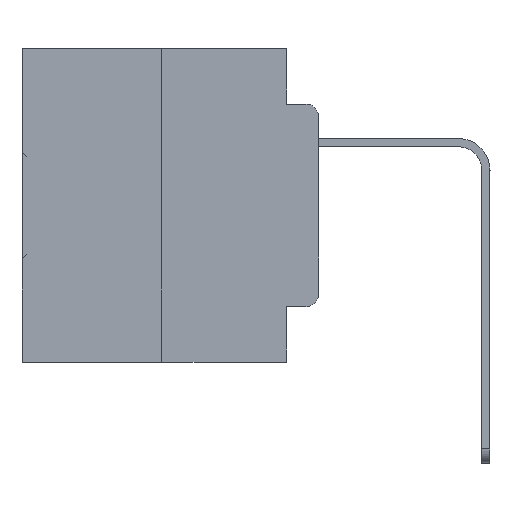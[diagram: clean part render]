
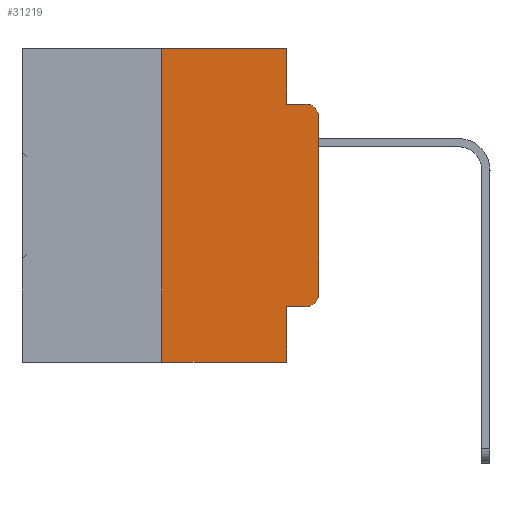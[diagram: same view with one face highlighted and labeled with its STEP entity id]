
A CAD part, left-side view. The second image highlights one B-rep face of the part: STEP entity #31219.
In plain terms, the highlighted planar face has unit normal (-1, 0, 0).
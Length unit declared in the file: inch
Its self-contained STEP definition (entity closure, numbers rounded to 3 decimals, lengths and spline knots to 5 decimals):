
#887 = ORIENTED_EDGE ( 'NONE', *, *, #29479, .F. ) ;
#1466 = DIRECTION ( 'NONE',  ( 0., 0., -1. ) ) ;
#1621 = AXIS2_PLACEMENT_3D ( 'NONE', #15515, #18575, #21191 ) ;
#1996 = EDGE_CURVE ( 'NONE', #19484, #26341, #17021, .T. ) ;
#2069 = DIRECTION ( 'NONE',  ( 0., -1., 0. ) ) ;
#2101 = DIRECTION ( 'NONE',  ( 0., 0., -1. ) ) ;
#4455 = DIRECTION ( 'NONE',  ( -1., 0., 0. ) ) ;
#4811 = FACE_OUTER_BOUND ( 'NONE', #15446, .T. ) ;
#5388 = DIRECTION ( 'NONE',  ( 0., -1., 0. ) ) ;
#5405 = EDGE_CURVE ( 'NONE', #26341, #24975, #33362, .T. ) ;
#5673 = VECTOR ( 'NONE', #28292, 39.37008 ) ;
#5837 = EDGE_CURVE ( 'NONE', #30265, #30139, #6894, .T. ) ;
#6894 = LINE ( 'NONE', #7854, #5673 ) ;
#7000 = DIRECTION ( 'NONE',  ( 0., 0., 1. ) ) ;
#7259 = VERTEX_POINT ( 'NONE', #8800 ) ;
#7507 = CARTESIAN_POINT ( 'NONE',  ( 0., 0.051, -0.4115 ) ) ;
#7854 = CARTESIAN_POINT ( 'NONE',  ( 0., 0.473, -0.5 ) ) ;
#8089 = CARTESIAN_POINT ( 'NONE',  ( 0., 0.02, -0.1085 ) ) ;
#8243 = CARTESIAN_POINT ( 'NONE',  ( 0., 0.051, -0.5 ) ) ;
#8558 = LINE ( 'NONE', #25778, #22320 ) ;
#8800 = CARTESIAN_POINT ( 'NONE',  ( 0., 0.051, -0.4115 ) ) ;
#9047 = EDGE_CURVE ( 'NONE', #29250, #19484, #24565, .T. ) ;
#9221 = ORIENTED_EDGE ( 'NONE', *, *, #23656, .F. ) ;
#9769 = ORIENTED_EDGE ( 'NONE', *, *, #24584, .F. ) ;
#9908 = DIRECTION ( 'NONE',  ( 0., 0., 1. ) ) ;
#10687 = AXIS2_PLACEMENT_3D ( 'NONE', #8089, #13526, #23230 ) ;
#11153 = ORIENTED_EDGE ( 'NONE', *, *, #20697, .T. ) ;
#12171 = VECTOR ( 'NONE', #5388, 39.37008 ) ;
#13526 = DIRECTION ( 'NONE',  ( -1., 0., 0. ) ) ;
#13672 = CARTESIAN_POINT ( 'NONE',  ( 0., 0.02, -0.0885 ) ) ;
#14201 = LINE ( 'NONE', #28673, #12171 ) ;
#14596 = VECTOR ( 'NONE', #9908, 39.37008 ) ;
#14891 = CARTESIAN_POINT ( 'NONE',  ( 0., 0., 0. ) ) ;
#15446 = EDGE_LOOP ( 'NONE', ( #18993, #32579, #9221, #16066, #15832, #9769, #26305, #887, #11153, #31463 ) ) ;
#15515 = CARTESIAN_POINT ( 'NONE',  ( 0., 0.473, 0. ) ) ;
#15832 = ORIENTED_EDGE ( 'NONE', *, *, #20690, .F. ) ;
#16066 = ORIENTED_EDGE ( 'NONE', *, *, #31467, .F. ) ;
#16459 = VECTOR ( 'NONE', #7000, 39.37008 ) ;
#16614 = CARTESIAN_POINT ( 'NONE',  ( 0., 0.02, -0.4115 ) ) ;
#16615 = VECTOR ( 'NONE', #33086, 39.37008 ) ;
#16809 = VERTEX_POINT ( 'NONE', #27671 ) ;
#16931 = VECTOR ( 'NONE', #1466, 39.37008 ) ;
#17021 = LINE ( 'NONE', #14891, #14596 ) ;
#17691 = DIRECTION ( 'NONE',  ( 0., 0., -1. ) ) ;
#18575 = DIRECTION ( 'NONE',  ( 1., 0., 0. ) ) ;
#18993 = ORIENTED_EDGE ( 'NONE', *, *, #1996, .T. ) ;
#19089 = CARTESIAN_POINT ( 'NONE',  ( 0., 0.25, -0.5 ) ) ;
#19484 = VERTEX_POINT ( 'NONE', #25956 ) ;
#20261 = LINE ( 'NONE', #7507, #16615 ) ;
#20279 = VERTEX_POINT ( 'NONE', #32003 ) ;
#20690 = EDGE_CURVE ( 'NONE', #16809, #27529, #14201, .T. ) ;
#20697 = EDGE_CURVE ( 'NONE', #7259, #29250, #20261, .T. ) ;
#21191 = DIRECTION ( 'NONE',  ( 0., 0., -1. ) ) ;
#22320 = VECTOR ( 'NONE', #2101, 39.37008 ) ;
#23230 = DIRECTION ( 'NONE',  ( 0., 0., -1. ) ) ;
#23656 = EDGE_CURVE ( 'NONE', #20279, #24975, #30086, .T. ) ;
#23787 = CARTESIAN_POINT ( 'NONE',  ( 0., 0.051, 0. ) ) ;
#23850 = LINE ( 'NONE', #32487, #16931 ) ;
#24565 = CIRCLE ( 'NONE', #33094, 0.02 ) ;
#24584 = EDGE_CURVE ( 'NONE', #30265, #16809, #29021, .T. ) ;
#24975 = VERTEX_POINT ( 'NONE', #13672 ) ;
#25778 = CARTESIAN_POINT ( 'NONE',  ( 0., 0.051, 0. ) ) ;
#25956 = CARTESIAN_POINT ( 'NONE',  ( 0., 0., -0.3915 ) ) ;
#26305 = ORIENTED_EDGE ( 'NONE', *, *, #5837, .T. ) ;
#26341 = VERTEX_POINT ( 'NONE', #29549 ) ;
#27256 = VECTOR ( 'NONE', #2069, 39.37008 ) ;
#27529 = VERTEX_POINT ( 'NONE', #23787 ) ;
#27671 = CARTESIAN_POINT ( 'NONE',  ( 0., 0.25, 0. ) ) ;
#28292 = DIRECTION ( 'NONE',  ( 0., -1., 0. ) ) ;
#28673 = CARTESIAN_POINT ( 'NONE',  ( 0., 0.473, 0. ) ) ;
#28863 = PLANE ( 'NONE',  #1621 ) ;
#29021 = LINE ( 'NONE', #33025, #16459 ) ;
#29250 = VERTEX_POINT ( 'NONE', #16614 ) ;
#29479 = EDGE_CURVE ( 'NONE', #7259, #30139, #8558, .T. ) ;
#29549 = CARTESIAN_POINT ( 'NONE',  ( 0., 0., -0.1085 ) ) ;
#30086 = LINE ( 'NONE', #32867, #27256 ) ;
#30139 = VERTEX_POINT ( 'NONE', #8243 ) ;
#30265 = VERTEX_POINT ( 'NONE', #19089 ) ;
#31219 = ADVANCED_FACE ( 'NONE', ( #4811 ), #28863, .F. ) ;
#31463 = ORIENTED_EDGE ( 'NONE', *, *, #9047, .T. ) ;
#31467 = EDGE_CURVE ( 'NONE', #27529, #20279, #23850, .T. ) ;
#32003 = CARTESIAN_POINT ( 'NONE',  ( 0., 0.051, -0.0885 ) ) ;
#32487 = CARTESIAN_POINT ( 'NONE',  ( 0., 0.051, 0. ) ) ;
#32579 = ORIENTED_EDGE ( 'NONE', *, *, #5405, .T. ) ;
#32867 = CARTESIAN_POINT ( 'NONE',  ( 0., 0.051, -0.0885 ) ) ;
#33025 = CARTESIAN_POINT ( 'NONE',  ( 0., 0.25, 0. ) ) ;
#33086 = DIRECTION ( 'NONE',  ( 0., -1., 0. ) ) ;
#33094 = AXIS2_PLACEMENT_3D ( 'NONE', #33210, #4455, #17691 ) ;
#33210 = CARTESIAN_POINT ( 'NONE',  ( 0., 0.02, -0.3915 ) ) ;
#33362 = CIRCLE ( 'NONE', #10687, 0.02 ) ;
